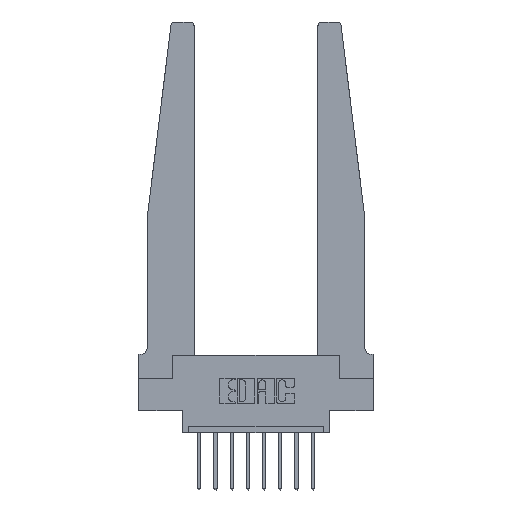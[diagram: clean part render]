
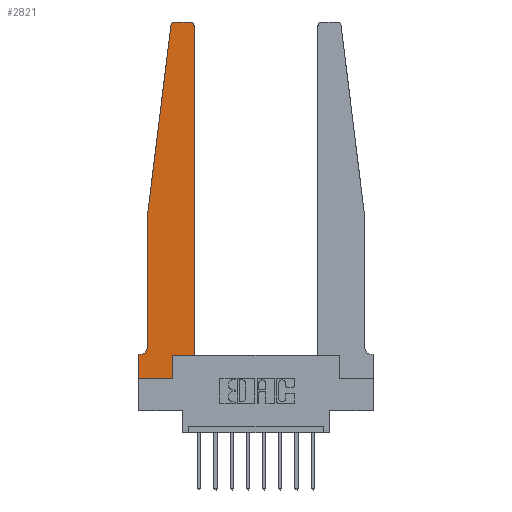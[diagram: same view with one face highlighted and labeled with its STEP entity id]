
A CAD part, top view. The second image highlights one B-rep face of the part: STEP entity #2821.
In plain terms, the highlighted planar face has unit normal (0, 0, 1).
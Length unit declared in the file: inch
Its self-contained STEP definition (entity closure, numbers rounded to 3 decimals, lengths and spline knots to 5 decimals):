
#143 = VERTEX_POINT ( 'NONE', #11292 ) ;
#164 = LINE ( 'NONE', #8290, #3269 ) ;
#183 = CARTESIAN_POINT ( 'NONE',  ( 0.2605, 0.18, 0.37 ) ) ;
#206 = ORIENTED_EDGE ( 'NONE', *, *, #3924, .T. ) ;
#605 = ORIENTED_EDGE ( 'NONE', *, *, #9509, .T. ) ;
#684 = CIRCLE ( 'NONE', #5976, 0.05 ) ;
#716 = EDGE_CURVE ( 'NONE', #6102, #830, #1467, .T. ) ;
#817 = PLANE ( 'NONE',  #6483 ) ;
#830 = VERTEX_POINT ( 'NONE', #5378 ) ;
#848 = VECTOR ( 'NONE', #3494, 39.37008 ) ;
#988 = DIRECTION ( 'NONE',  ( 0., 0., 1. ) ) ;
#1057 = CARTESIAN_POINT ( 'NONE',  ( 0.395, 2.72, 0.37 ) ) ;
#1196 = ORIENTED_EDGE ( 'NONE', *, *, #8133, .T. ) ;
#1365 = CARTESIAN_POINT ( 'NONE',  ( 0.065, 1.25, 0.37 ) ) ;
#1435 = ORIENTED_EDGE ( 'NONE', *, *, #5677, .T. ) ;
#1467 = LINE ( 'NONE', #183, #12214 ) ;
#1838 = ORIENTED_EDGE ( 'NONE', *, *, #6653, .T. ) ;
#1977 = LINE ( 'NONE', #13415, #13556 ) ;
#2109 = ORIENTED_EDGE ( 'NONE', *, *, #11876, .T. ) ;
#2364 = DIRECTION ( 'NONE',  ( -1., 0., 0. ) ) ;
#2500 = CARTESIAN_POINT ( 'NONE',  ( 0.425, 0.18, 0.37 ) ) ;
#2652 = VECTOR ( 'NONE', #14875, 39.37008 ) ;
#2821 = ADVANCED_FACE ( 'NONE', ( #3389 ), #817, .T. ) ;
#2903 = DIRECTION ( 'NONE',  ( -1., 0., 0. ) ) ;
#3055 = CARTESIAN_POINT ( 'NONE',  ( 0.2605, 0., 0.37 ) ) ;
#3208 = VECTOR ( 'NONE', #4415, 39.37008 ) ;
#3269 = VECTOR ( 'NONE', #2364, 39.37008 ) ;
#3389 = FACE_OUTER_BOUND ( 'NONE', #12087, .T. ) ;
#3494 = DIRECTION ( 'NONE',  ( -1., 0., 0. ) ) ;
#3643 = LINE ( 'NONE', #2500, #8614 ) ;
#3721 = VERTEX_POINT ( 'NONE', #13029 ) ;
#3924 = EDGE_CURVE ( 'NONE', #14518, #6102, #10001, .T. ) ;
#3963 = CARTESIAN_POINT ( 'NONE',  ( 0.015, 0.2375, 0.37 ) ) ;
#4307 = VERTEX_POINT ( 'NONE', #13160 ) ;
#4363 = VERTEX_POINT ( 'NONE', #5629 ) ;
#4415 = DIRECTION ( 'NONE',  ( 0., -1., 0. ) ) ;
#5174 = ORIENTED_EDGE ( 'NONE', *, *, #9378, .T. ) ;
#5335 = CIRCLE ( 'NONE', #9158, 0.03 ) ;
#5378 = CARTESIAN_POINT ( 'NONE',  ( 0.2605, 0.18, 0.37 ) ) ;
#5497 = ORIENTED_EDGE ( 'NONE', *, *, #716, .T. ) ;
#5501 = CARTESIAN_POINT ( 'NONE',  ( 0., 0.1875, 0.37 ) ) ;
#5542 = CARTESIAN_POINT ( 'NONE',  ( 0., 0.1875, 0.37 ) ) ;
#5578 = DIRECTION ( 'NONE',  ( 1., 0., 0. ) ) ;
#5629 = CARTESIAN_POINT ( 'NONE',  ( 0.24675, 2.72367, 0.37 ) ) ;
#5677 = EDGE_CURVE ( 'NONE', #6415, #9928, #13676, .T. ) ;
#5701 = CARTESIAN_POINT ( 'NONE',  ( 0.395, 2.75, 0.37 ) ) ;
#5890 = LINE ( 'NONE', #12825, #848 ) ;
#5976 = AXIS2_PLACEMENT_3D ( 'NONE', #3963, #6438, #2903 ) ;
#6102 = VERTEX_POINT ( 'NONE', #3055 ) ;
#6259 = LINE ( 'NONE', #10933, #13843 ) ;
#6267 = CARTESIAN_POINT ( 'NONE',  ( 0.27653, 2.75, 0.37 ) ) ;
#6367 = VERTEX_POINT ( 'NONE', #5542 ) ;
#6407 = DIRECTION ( 'NONE',  ( -0.122, -0.992, 0. ) ) ;
#6415 = VERTEX_POINT ( 'NONE', #1365 ) ;
#6425 = DIRECTION ( 'NONE',  ( 0., 1., 0. ) ) ;
#6438 = DIRECTION ( 'NONE',  ( 0., 0., -1. ) ) ;
#6483 = AXIS2_PLACEMENT_3D ( 'NONE', #5501, #11141, #11360 ) ;
#6525 = CARTESIAN_POINT ( 'NONE',  ( 0., 0., 0.37 ) ) ;
#6653 = EDGE_CURVE ( 'NONE', #143, #7387, #5335, .T. ) ;
#7387 = VERTEX_POINT ( 'NONE', #5701 ) ;
#7618 = CARTESIAN_POINT ( 'NONE',  ( 0.27653, 2.72, 0.37 ) ) ;
#7703 = DIRECTION ( 'NONE',  ( 0., 0., 1. ) ) ;
#7850 = EDGE_CURVE ( 'NONE', #6367, #14518, #7932, .T. ) ;
#7932 = LINE ( 'NONE', #14717, #3208 ) ;
#8049 = CIRCLE ( 'NONE', #9503, 0.03 ) ;
#8133 = EDGE_CURVE ( 'NONE', #4363, #6415, #1977, .T. ) ;
#8290 = CARTESIAN_POINT ( 'NONE',  ( 0.25, 2.75, 0.37 ) ) ;
#8614 = VECTOR ( 'NONE', #13055, 39.37008 ) ;
#9134 = EDGE_CURVE ( 'NONE', #7387, #11136, #164, .T. ) ;
#9158 = AXIS2_PLACEMENT_3D ( 'NONE', #1057, #988, #14840 ) ;
#9378 = EDGE_CURVE ( 'NONE', #11136, #4363, #8049, .T. ) ;
#9426 = ORIENTED_EDGE ( 'NONE', *, *, #9678, .T. ) ;
#9503 = AXIS2_PLACEMENT_3D ( 'NONE', #7618, #7703, #12458 ) ;
#9509 = EDGE_CURVE ( 'NONE', #4307, #6367, #5890, .T. ) ;
#9678 = EDGE_CURVE ( 'NONE', #3721, #143, #6259, .T. ) ;
#9872 = ORIENTED_EDGE ( 'NONE', *, *, #12296, .T. ) ;
#9928 = VERTEX_POINT ( 'NONE', #13256 ) ;
#10001 = LINE ( 'NONE', #12647, #10780 ) ;
#10780 = VECTOR ( 'NONE', #5578, 39.37008 ) ;
#10933 = CARTESIAN_POINT ( 'NONE',  ( 0.425, 0.18, 0.37 ) ) ;
#11136 = VERTEX_POINT ( 'NONE', #6267 ) ;
#11141 = DIRECTION ( 'NONE',  ( 0., 0., 1. ) ) ;
#11292 = CARTESIAN_POINT ( 'NONE',  ( 0.425, 2.72, 0.37 ) ) ;
#11360 = DIRECTION ( 'NONE',  ( 1., 0., 0. ) ) ;
#11876 = EDGE_CURVE ( 'NONE', #9928, #4307, #684, .T. ) ;
#12087 = EDGE_LOOP ( 'NONE', ( #14080, #5174, #1196, #1435, #2109, #605, #14250, #206, #5497, #9872, #9426, #1838 ) ) ;
#12214 = VECTOR ( 'NONE', #6425, 39.37008 ) ;
#12296 = EDGE_CURVE ( 'NONE', #830, #3721, #3643, .T. ) ;
#12458 = DIRECTION ( 'NONE',  ( 1., 0., 0. ) ) ;
#12564 = CARTESIAN_POINT ( 'NONE',  ( 0.065, 1.25, 0.37 ) ) ;
#12647 = CARTESIAN_POINT ( 'NONE',  ( 0., 0., 0.37 ) ) ;
#12825 = CARTESIAN_POINT ( 'NONE',  ( 0.065, 0.1875, 0.37 ) ) ;
#13029 = CARTESIAN_POINT ( 'NONE',  ( 0.425, 0.18, 0.37 ) ) ;
#13055 = DIRECTION ( 'NONE',  ( 1., 0., 0. ) ) ;
#13160 = CARTESIAN_POINT ( 'NONE',  ( 0.015, 0.1875, 0.37 ) ) ;
#13256 = CARTESIAN_POINT ( 'NONE',  ( 0.065, 0.2375, 0.37 ) ) ;
#13415 = CARTESIAN_POINT ( 'NONE',  ( 0.065, 1.25, 0.37 ) ) ;
#13556 = VECTOR ( 'NONE', #6407, 39.37008 ) ;
#13676 = LINE ( 'NONE', #12564, #2652 ) ;
#13843 = VECTOR ( 'NONE', #14077, 39.37008 ) ;
#14077 = DIRECTION ( 'NONE',  ( 0., 1., 0. ) ) ;
#14080 = ORIENTED_EDGE ( 'NONE', *, *, #9134, .T. ) ;
#14250 = ORIENTED_EDGE ( 'NONE', *, *, #7850, .T. ) ;
#14518 = VERTEX_POINT ( 'NONE', #6525 ) ;
#14717 = CARTESIAN_POINT ( 'NONE',  ( 0., 0., 0.37 ) ) ;
#14840 = DIRECTION ( 'NONE',  ( 1., 0., 0. ) ) ;
#14875 = DIRECTION ( 'NONE',  ( 0., -1., 0. ) ) ;
